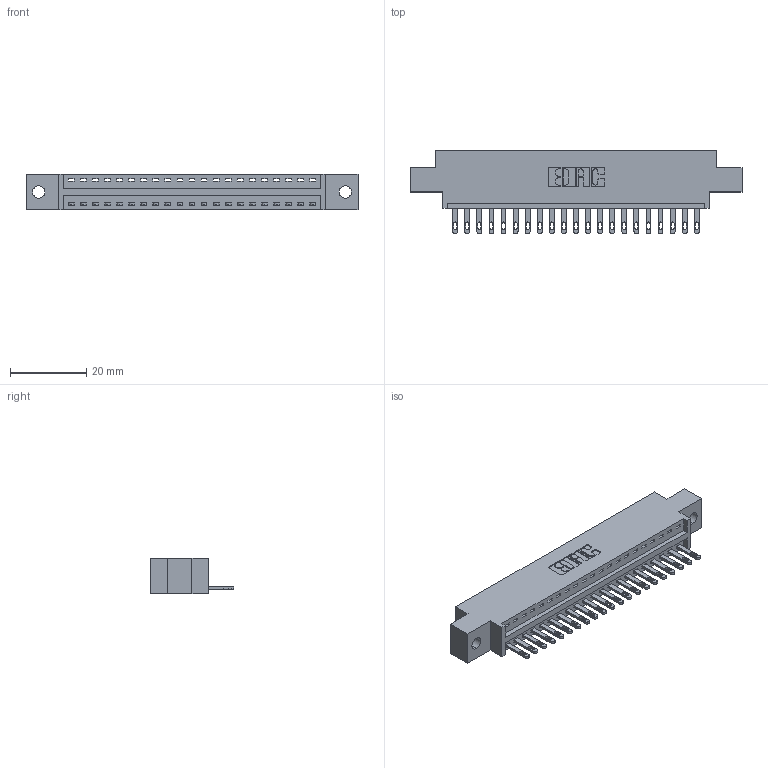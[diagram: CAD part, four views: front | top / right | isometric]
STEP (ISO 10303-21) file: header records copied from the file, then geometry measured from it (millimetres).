
FILE_DESCRIPTION (( 'STEP AP203' ), '1' );
FILE_NAME ('896-021-500-602.STEP', '2021-07-27T16:48:01', ( '' ), ( '' ), 'SwSTEP 2.0', 'SolidWorks 2020', '' );
FILE_SCHEMA (( 'CONFIG_CONTROL_DESIGN' ));
Length unit declared in the file: inch
Products named in the file (3): 846 Part_0.170 Offset - 0.128 Dia; 896-021-500-602; 345-292-001_345-293-100
Assembly tree (22 placements, depth 2):
  896-021-500-602
    846 Part_0.170 Offset - 0.128 Dia
    345-292-001_345-293-100  x21
Bounding box: 87.25 x 21.84 x 9.4 mm (x, y, z)
Volume: 8028.7 mm3; surface area: 9746.2 mm2
Topology: 22 solids, 22 shells, 1260 faces, 3869 edges, 2578 vertices
Faces by surface type: plane 794, cylinder 466
Entity records: 15925 total; most frequent: CARTESIAN_POINT 2743, ORIENTED_EDGE 2698, DIRECTION 2447, EDGE_CURVE 1349, VECTOR 1129, LINE 1129, VERTEX_POINT 898, AXIS2_PLACEMENT_3D 659
